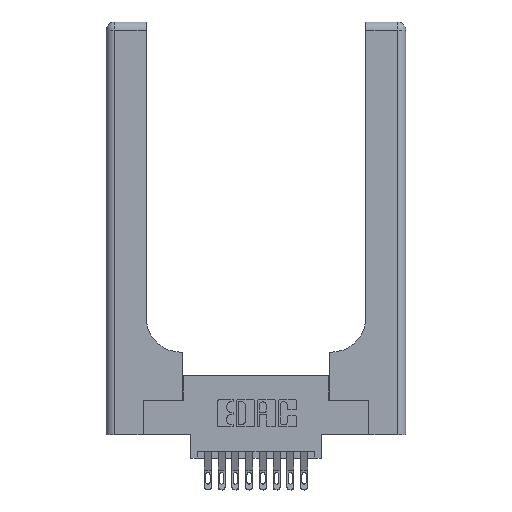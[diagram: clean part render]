
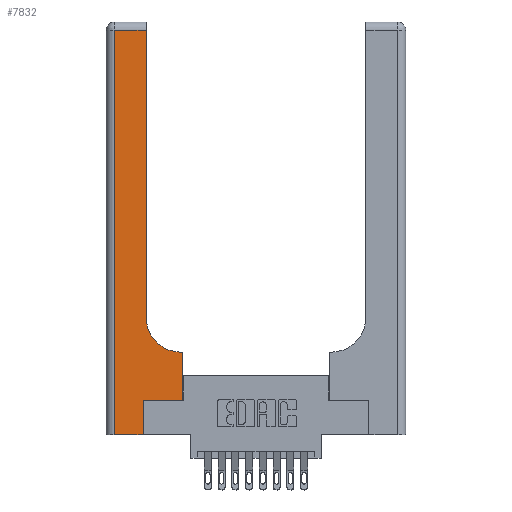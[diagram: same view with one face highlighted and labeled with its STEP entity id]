
A CAD part, top view. The second image highlights one B-rep face of the part: STEP entity #7832.
In plain terms, the highlighted planar face has unit normal (0, 0, 1).
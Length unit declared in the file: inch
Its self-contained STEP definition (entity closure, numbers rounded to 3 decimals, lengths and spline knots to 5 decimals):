
#13 = VERTEX_POINT ( 'NONE', #223 ) ;
#223 = CARTESIAN_POINT ( 'NONE',  ( 0.2915, 2.94, 0.37 ) ) ;
#341 = DIRECTION ( 'NONE',  ( -1., 0., 0. ) ) ;
#759 = VERTEX_POINT ( 'NONE', #11262 ) ;
#790 = DIRECTION ( 'NONE',  ( -1., 0., 0. ) ) ;
#1613 = LINE ( 'NONE', #15040, #8018 ) ;
#1688 = ORIENTED_EDGE ( 'NONE', *, *, #3081, .T. ) ;
#1692 = AXIS2_PLACEMENT_3D ( 'NONE', #16497, #16359, #16264 ) ;
#1704 = CARTESIAN_POINT ( 'NONE',  ( 0.2915, 0.6, 0.37 ) ) ;
#2250 = CIRCLE ( 'NONE', #1692, 0.25 ) ;
#2293 = VERTEX_POINT ( 'NONE', #9532 ) ;
#2777 = CARTESIAN_POINT ( 'NONE',  ( 0.2915, 3., 0.37 ) ) ;
#2803 = VECTOR ( 'NONE', #14124, 39.37008 ) ;
#3013 = VECTOR ( 'NONE', #15182, 39.37008 ) ;
#3081 = EDGE_CURVE ( 'NONE', #10559, #10449, #1613, .T. ) ;
#3170 = CARTESIAN_POINT ( 'NONE',  ( 0.5585, 0.25, 0.37 ) ) ;
#3311 = EDGE_CURVE ( 'NONE', #9796, #4638, #2250, .T. ) ;
#3480 = DIRECTION ( 'NONE',  ( 0., 1., 0. ) ) ;
#3717 = VECTOR ( 'NONE', #341, 39.37008 ) ;
#4004 = AXIS2_PLACEMENT_3D ( 'NONE', #9704, #8468, #790 ) ;
#4067 = VERTEX_POINT ( 'NONE', #4156 ) ;
#4135 = CARTESIAN_POINT ( 'NONE',  ( 0.2915, 0.85, 0.37 ) ) ;
#4137 = FACE_OUTER_BOUND ( 'NONE', #9991, .T. ) ;
#4156 = CARTESIAN_POINT ( 'NONE',  ( 0.06, 2.94, 0.37 ) ) ;
#4638 = VERTEX_POINT ( 'NONE', #4135 ) ;
#4707 = CARTESIAN_POINT ( 'NONE',  ( 0.5415, 0.6, 0.37 ) ) ;
#4742 = CARTESIAN_POINT ( 'NONE',  ( 0.269, 0.25, 0.37 ) ) ;
#4760 = VECTOR ( 'NONE', #15658, 39.37008 ) ;
#5018 = CARTESIAN_POINT ( 'NONE',  ( 0.269, 0.25, 0.37 ) ) ;
#5058 = EDGE_CURVE ( 'NONE', #13, #4067, #14528, .T. ) ;
#5854 = ORIENTED_EDGE ( 'NONE', *, *, #15938, .T. ) ;
#6021 = DIRECTION ( 'NONE',  ( 1., 0., 0. ) ) ;
#6229 = DIRECTION ( 'NONE',  ( -1., 0., 0. ) ) ;
#6338 = ORIENTED_EDGE ( 'NONE', *, *, #3311, .T. ) ;
#6403 = CARTESIAN_POINT ( 'NONE',  ( 0.06, 3., 0.37 ) ) ;
#6470 = EDGE_CURVE ( 'NONE', #759, #10559, #15265, .T. ) ;
#7591 = VECTOR ( 'NONE', #3480, 39.37008 ) ;
#7832 = ADVANCED_FACE ( 'NONE', ( #4137 ), #15983, .F. ) ;
#7986 = LINE ( 'NONE', #16065, #7591 ) ;
#8018 = VECTOR ( 'NONE', #14897, 39.37008 ) ;
#8140 = ORIENTED_EDGE ( 'NONE', *, *, #8342, .T. ) ;
#8279 = ORIENTED_EDGE ( 'NONE', *, *, #15195, .T. ) ;
#8295 = ORIENTED_EDGE ( 'NONE', *, *, #15598, .T. ) ;
#8342 = EDGE_CURVE ( 'NONE', #2293, #9796, #13850, .T. ) ;
#8465 = ORIENTED_EDGE ( 'NONE', *, *, #5058, .T. ) ;
#8468 = DIRECTION ( 'NONE',  ( 0., 0., -1. ) ) ;
#9161 = LINE ( 'NONE', #2777, #2803 ) ;
#9343 = CARTESIAN_POINT ( 'NONE',  ( 0., 0., 0.37 ) ) ;
#9532 = CARTESIAN_POINT ( 'NONE',  ( 0.5585, 0.6, 0.37 ) ) ;
#9646 = VERTEX_POINT ( 'NONE', #3170 ) ;
#9704 = CARTESIAN_POINT ( 'NONE',  ( 0., 3., 0.37 ) ) ;
#9796 = VERTEX_POINT ( 'NONE', #4707 ) ;
#9991 = EDGE_LOOP ( 'NONE', ( #5854, #8465, #8279, #15967, #1688, #13021, #8295, #8140, #6338 ) ) ;
#10188 = LINE ( 'NONE', #6403, #3013 ) ;
#10325 = EDGE_CURVE ( 'NONE', #10449, #9646, #10912, .T. ) ;
#10449 = VERTEX_POINT ( 'NONE', #5018 ) ;
#10559 = VERTEX_POINT ( 'NONE', #14061 ) ;
#10912 = LINE ( 'NONE', #4742, #13860 ) ;
#11180 = VECTOR ( 'NONE', #6229, 39.37008 ) ;
#11262 = CARTESIAN_POINT ( 'NONE',  ( 0.06, 0., 0.37 ) ) ;
#13021 = ORIENTED_EDGE ( 'NONE', *, *, #10325, .T. ) ;
#13850 = LINE ( 'NONE', #1704, #3717 ) ;
#13860 = VECTOR ( 'NONE', #6021, 39.37008 ) ;
#14061 = CARTESIAN_POINT ( 'NONE',  ( 0.269, 0., 0.37 ) ) ;
#14124 = DIRECTION ( 'NONE',  ( 0., 1., 0. ) ) ;
#14528 = LINE ( 'NONE', #16259, #11180 ) ;
#14897 = DIRECTION ( 'NONE',  ( 0., 1., 0. ) ) ;
#15040 = CARTESIAN_POINT ( 'NONE',  ( 0.269, 0., 0.37 ) ) ;
#15182 = DIRECTION ( 'NONE',  ( 0., -1., 0. ) ) ;
#15195 = EDGE_CURVE ( 'NONE', #4067, #759, #10188, .T. ) ;
#15265 = LINE ( 'NONE', #9343, #4760 ) ;
#15598 = EDGE_CURVE ( 'NONE', #9646, #2293, #7986, .T. ) ;
#15658 = DIRECTION ( 'NONE',  ( 1., 0., 0. ) ) ;
#15938 = EDGE_CURVE ( 'NONE', #4638, #13, #9161, .T. ) ;
#15967 = ORIENTED_EDGE ( 'NONE', *, *, #6470, .T. ) ;
#15983 = PLANE ( 'NONE',  #4004 ) ;
#16065 = CARTESIAN_POINT ( 'NONE',  ( 0.5585, 0.25, 0.37 ) ) ;
#16259 = CARTESIAN_POINT ( 'NONE',  ( 0., 2.94, 0.37 ) ) ;
#16264 = DIRECTION ( 'NONE',  ( 1., 0., 0. ) ) ;
#16359 = DIRECTION ( 'NONE',  ( 0., 0., -1. ) ) ;
#16497 = CARTESIAN_POINT ( 'NONE',  ( 0.5415, 0.85, 0.37 ) ) ;
